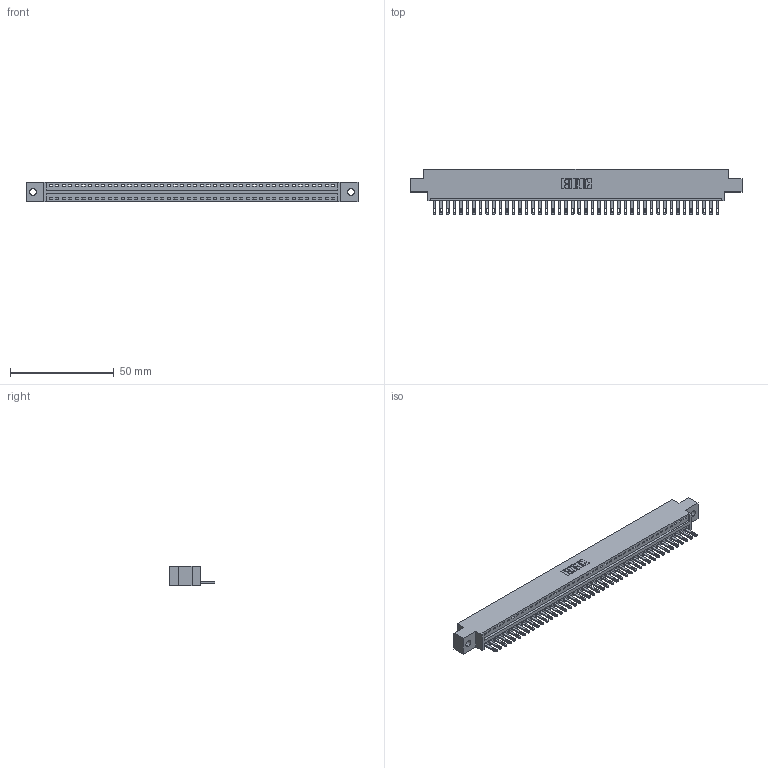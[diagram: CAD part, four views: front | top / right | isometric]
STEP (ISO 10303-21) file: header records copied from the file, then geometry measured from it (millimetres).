
FILE_DESCRIPTION (( 'STEP AP203' ), '1' );
FILE_NAME ('896-044-500-602.STEP', '2021-07-27T22:06:21', ( '' ), ( '' ), 'SwSTEP 2.0', 'SolidWorks 2020', '' );
FILE_SCHEMA (( 'CONFIG_CONTROL_DESIGN' ));
Length unit declared in the file: inch
Products named in the file (3): 345-292-001_345-293-100; 846 Part_0.170 Offset - 0.128 Dia; 896-044-500-602
Assembly tree (45 placements, depth 2):
  896-044-500-602
    846 Part_0.170 Offset - 0.128 Dia
    345-292-001_345-293-100  x44
Bounding box: 160.27 x 21.84 x 9.4 mm (x, y, z)
Volume: 15191.5 mm3; surface area: 19000.6 mm2
Topology: 45 solids, 45 shells, 2502 faces, 7733 edges, 5154 vertices
Faces by surface type: plane 1576, cylinder 926
Entity records: 27103 total; most frequent: CARTESIAN_POINT 4652, ORIENTED_EDGE 4630, DIRECTION 4103, EDGE_CURVE 2315, LINE 2003, VECTOR 2003, VERTEX_POINT 1542, AXIS2_PLACEMENT_3D 1050
